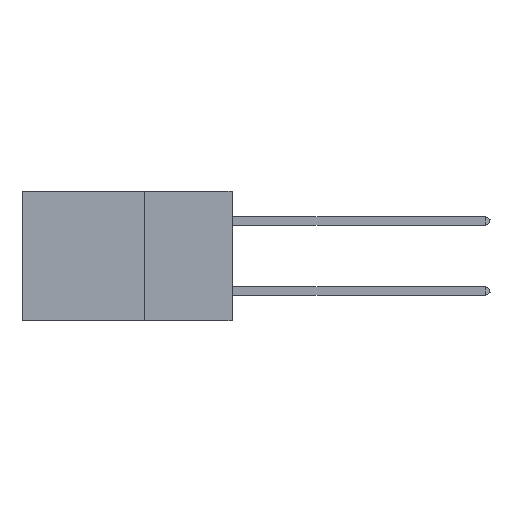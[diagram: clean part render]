
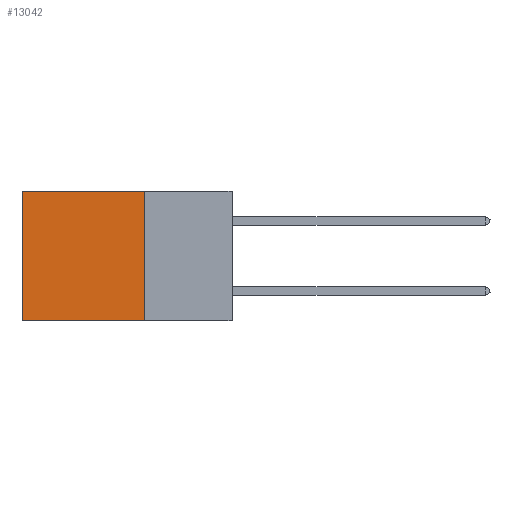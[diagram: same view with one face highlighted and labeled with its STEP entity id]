
A CAD part, left-side view. The second image highlights one B-rep face of the part: STEP entity #13042.
In plain terms, the highlighted planar face has unit normal (-1, 0, 0).
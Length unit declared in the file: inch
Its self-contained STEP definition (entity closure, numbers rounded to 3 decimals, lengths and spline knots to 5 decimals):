
#1411 = LINE ( 'NONE', #6221, #15185 ) ;
#2841 = VECTOR ( 'NONE', #42434, 39.37008 ) ;
#3909 = FACE_OUTER_BOUND ( 'NONE', #29247, .T. ) ;
#6073 = PLANE ( 'NONE',  #18017 ) ;
#6221 = CARTESIAN_POINT ( 'NONE',  ( 0.2875, 0.6, 0. ) ) ;
#9800 = EDGE_CURVE ( 'NONE', #20558, #30480, #1411, .T. ) ;
#10329 = CARTESIAN_POINT ( 'NONE',  ( 0.2875, 0.6, 0. ) ) ;
#10964 = VERTEX_POINT ( 'NONE', #30279 ) ;
#12815 = CARTESIAN_POINT ( 'NONE',  ( 0.2875, 0.25, 0. ) ) ;
#13042 = ADVANCED_FACE ( 'NONE', ( #3909 ), #6073, .F. ) ;
#14105 = LINE ( 'NONE', #17437, #38172 ) ;
#15185 = VECTOR ( 'NONE', #37418, 39.37008 ) ;
#16227 = DIRECTION ( 'NONE',  ( 1., 0., 0. ) ) ;
#17437 = CARTESIAN_POINT ( 'NONE',  ( 0.2875, 0.25, -0.37 ) ) ;
#18017 = AXIS2_PLACEMENT_3D ( 'NONE', #39868, #16227, #40644 ) ;
#18106 = CARTESIAN_POINT ( 'NONE',  ( 0.2875, 0.6, -0.37 ) ) ;
#20558 = VERTEX_POINT ( 'NONE', #10329 ) ;
#21503 = ORIENTED_EDGE ( 'NONE', *, *, #42186, .F. ) ;
#21810 = VECTOR ( 'NONE', #41614, 39.37008 ) ;
#23354 = ORIENTED_EDGE ( 'NONE', *, *, #9800, .T. ) ;
#26528 = VERTEX_POINT ( 'NONE', #12815 ) ;
#29247 = EDGE_LOOP ( 'NONE', ( #23354, #42135, #21503, #31618 ) ) ;
#30279 = CARTESIAN_POINT ( 'NONE',  ( 0.2875, 0.25, -0.37 ) ) ;
#30480 = VERTEX_POINT ( 'NONE', #18106 ) ;
#31618 = ORIENTED_EDGE ( 'NONE', *, *, #38148, .T. ) ;
#31720 = CARTESIAN_POINT ( 'NONE',  ( 0.2875, 0.25, 0. ) ) ;
#32379 = LINE ( 'NONE', #31720, #2841 ) ;
#37418 = DIRECTION ( 'NONE',  ( 0., 0., -1. ) ) ;
#38148 = EDGE_CURVE ( 'NONE', #26528, #20558, #32379, .T. ) ;
#38172 = VECTOR ( 'NONE', #42299, 39.37008 ) ;
#39868 = CARTESIAN_POINT ( 'NONE',  ( 0.2875, 0.25, 0. ) ) ;
#40624 = EDGE_CURVE ( 'NONE', #10964, #30480, #14105, .T. ) ;
#40644 = DIRECTION ( 'NONE',  ( 0., 0., -1. ) ) ;
#41469 = CARTESIAN_POINT ( 'NONE',  ( 0.2875, 0.25, 0. ) ) ;
#41614 = DIRECTION ( 'NONE',  ( 0., 0., -1. ) ) ;
#42135 = ORIENTED_EDGE ( 'NONE', *, *, #40624, .F. ) ;
#42186 = EDGE_CURVE ( 'NONE', #26528, #10964, #43718, .T. ) ;
#42299 = DIRECTION ( 'NONE',  ( 0., 1., 0. ) ) ;
#42434 = DIRECTION ( 'NONE',  ( 0., 1., 0. ) ) ;
#43718 = LINE ( 'NONE', #41469, #21810 ) ;
